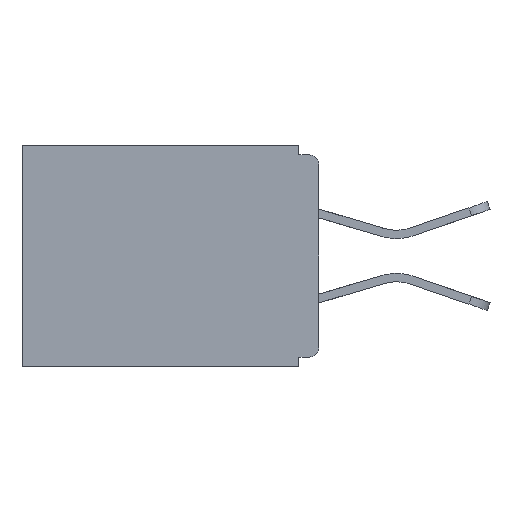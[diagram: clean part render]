
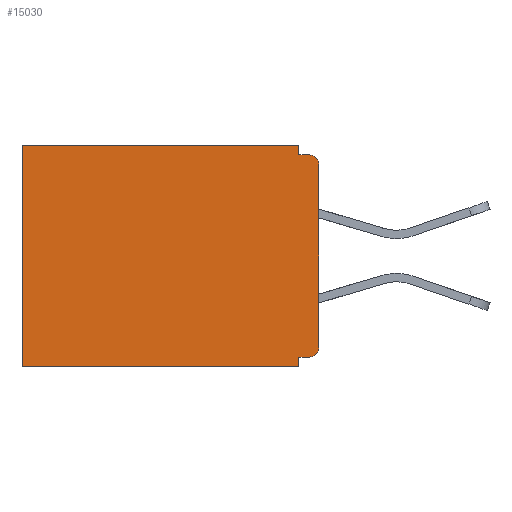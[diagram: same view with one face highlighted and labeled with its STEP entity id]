
A CAD part, left-side view. The second image highlights one B-rep face of the part: STEP entity #15030.
In plain terms, the highlighted planar face has unit normal (-1, 0, 0).
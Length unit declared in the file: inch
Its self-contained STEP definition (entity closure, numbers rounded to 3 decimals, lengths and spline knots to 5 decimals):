
#72 = VERTEX_POINT ( 'NONE', #19575 ) ;
#88 = DIRECTION ( 'NONE',  ( 0., 0., -1. ) ) ;
#672 = VECTOR ( 'NONE', #1396, 39.37008 ) ;
#871 = EDGE_CURVE ( 'NONE', #8522, #17490, #8414, .T. ) ;
#1396 = DIRECTION ( 'NONE',  ( 0., 0., -1. ) ) ;
#1463 = EDGE_CURVE ( 'NONE', #14093, #8041, #18573, .T. ) ;
#1473 = DIRECTION ( 'NONE',  ( 0., -1., 0. ) ) ;
#1577 = DIRECTION ( 'NONE',  ( 0., 0., -1. ) ) ;
#2273 = LINE ( 'NONE', #14384, #13811 ) ;
#2926 = EDGE_CURVE ( 'NONE', #14093, #8343, #18223, .T. ) ;
#3055 = ORIENTED_EDGE ( 'NONE', *, *, #6588, .T. ) ;
#3186 = VERTEX_POINT ( 'NONE', #16724 ) ;
#3974 = CARTESIAN_POINT ( 'NONE',  ( 0.298, 0.015, -0.328 ) ) ;
#4785 = ORIENTED_EDGE ( 'NONE', *, *, #9442, .F. ) ;
#4789 = DIRECTION ( 'NONE',  ( -1., 0., 0. ) ) ;
#4976 = CARTESIAN_POINT ( 'NONE',  ( 0.298, 0.031, -0.343 ) ) ;
#5769 = ORIENTED_EDGE ( 'NONE', *, *, #2926, .T. ) ;
#6076 = CARTESIAN_POINT ( 'NONE',  ( 0.298, 0., -0.328 ) ) ;
#6103 = CARTESIAN_POINT ( 'NONE',  ( 0.298, 0.015, -0.03 ) ) ;
#6588 = EDGE_CURVE ( 'NONE', #8075, #17490, #7877, .T. ) ;
#6614 = PLANE ( 'NONE',  #16510 ) ;
#6828 = ORIENTED_EDGE ( 'NONE', *, *, #19921, .T. ) ;
#6858 = LINE ( 'NONE', #13141, #7121 ) ;
#6919 = ORIENTED_EDGE ( 'NONE', *, *, #17527, .T. ) ;
#6967 = CARTESIAN_POINT ( 'NONE',  ( 0.298, 0., 0. ) ) ;
#7121 = VECTOR ( 'NONE', #1473, 39.37008 ) ;
#7652 = VERTEX_POINT ( 'NONE', #3974 ) ;
#7800 = DIRECTION ( 'NONE',  ( 0., 1., 0. ) ) ;
#7863 = VECTOR ( 'NONE', #19016, 39.37008 ) ;
#7877 = LINE ( 'NONE', #13534, #20760 ) ;
#8041 = VERTEX_POINT ( 'NONE', #13827 ) ;
#8075 = VERTEX_POINT ( 'NONE', #15954 ) ;
#8081 = CIRCLE ( 'NONE', #19873, 0.015 ) ;
#8231 = VECTOR ( 'NONE', #88, 39.37008 ) ;
#8343 = VERTEX_POINT ( 'NONE', #18941 ) ;
#8414 = LINE ( 'NONE', #17519, #7863 ) ;
#8522 = VERTEX_POINT ( 'NONE', #20768 ) ;
#9442 = EDGE_CURVE ( 'NONE', #9648, #8522, #17628, .T. ) ;
#9483 = LINE ( 'NONE', #6076, #13396 ) ;
#9648 = VERTEX_POINT ( 'NONE', #9981 ) ;
#9981 = CARTESIAN_POINT ( 'NONE',  ( 0.298, 0.031, -0.328 ) ) ;
#9983 = DIRECTION ( 'NONE',  ( 1., 0., 0. ) ) ;
#10261 = ORIENTED_EDGE ( 'NONE', *, *, #871, .F. ) ;
#10320 = EDGE_CURVE ( 'NONE', #7652, #9648, #9483, .T. ) ;
#10984 = ORIENTED_EDGE ( 'NONE', *, *, #16417, .F. ) ;
#11588 = FACE_OUTER_BOUND ( 'NONE', #12379, .T. ) ;
#11748 = CARTESIAN_POINT ( 'NONE',  ( 0.298, 0.015, -0.313 ) ) ;
#12283 = DIRECTION ( 'NONE',  ( 0., 0., -1. ) ) ;
#12379 = EDGE_LOOP ( 'NONE', ( #5769, #10984, #19087, #6919, #3055, #10261, #4785, #20620, #6828, #14695 ) ) ;
#12833 = DIRECTION ( 'NONE',  ( 0., 0., -1. ) ) ;
#13141 = CARTESIAN_POINT ( 'NONE',  ( 0.298, 0., -0.015 ) ) ;
#13396 = VECTOR ( 'NONE', #7800, 39.37008 ) ;
#13534 = CARTESIAN_POINT ( 'NONE',  ( 0.298, 0.46, 0. ) ) ;
#13811 = VECTOR ( 'NONE', #12833, 39.37008 ) ;
#13827 = CARTESIAN_POINT ( 'NONE',  ( 0.298, 0., -0.313 ) ) ;
#14093 = VERTEX_POINT ( 'NONE', #19792 ) ;
#14277 = AXIS2_PLACEMENT_3D ( 'NONE', #6103, #19577, #21236 ) ;
#14384 = CARTESIAN_POINT ( 'NONE',  ( 0.298, 0.031, -0.343 ) ) ;
#14695 = ORIENTED_EDGE ( 'NONE', *, *, #1463, .F. ) ;
#15030 = ADVANCED_FACE ( 'NONE', ( #11588 ), #6614, .F. ) ;
#15183 = LINE ( 'NONE', #6967, #21498 ) ;
#15310 = CARTESIAN_POINT ( 'NONE',  ( 0.298, 0.46, -0.343 ) ) ;
#15954 = CARTESIAN_POINT ( 'NONE',  ( 0.298, 0.46, 0. ) ) ;
#16344 = CARTESIAN_POINT ( 'NONE',  ( 0.298, 0., 0. ) ) ;
#16417 = EDGE_CURVE ( 'NONE', #72, #8343, #6858, .T. ) ;
#16510 = AXIS2_PLACEMENT_3D ( 'NONE', #18333, #9983, #1577 ) ;
#16539 = DIRECTION ( 'NONE',  ( 0., 0., -1. ) ) ;
#16724 = CARTESIAN_POINT ( 'NONE',  ( 0.298, 0.031, 0. ) ) ;
#17490 = VERTEX_POINT ( 'NONE', #15310 ) ;
#17519 = CARTESIAN_POINT ( 'NONE',  ( 0.298, 0., -0.343 ) ) ;
#17527 = EDGE_CURVE ( 'NONE', #3186, #8075, #15183, .T. ) ;
#17628 = LINE ( 'NONE', #4976, #8231 ) ;
#18223 = CIRCLE ( 'NONE', #14277, 0.015 ) ;
#18333 = CARTESIAN_POINT ( 'NONE',  ( 0.298, 0., 0. ) ) ;
#18515 = DIRECTION ( 'NONE',  ( 0., 1., 0. ) ) ;
#18573 = LINE ( 'NONE', #16344, #672 ) ;
#18758 = EDGE_CURVE ( 'NONE', #3186, #72, #2273, .T. ) ;
#18941 = CARTESIAN_POINT ( 'NONE',  ( 0.298, 0.015, -0.015 ) ) ;
#19016 = DIRECTION ( 'NONE',  ( 0., 1., 0. ) ) ;
#19087 = ORIENTED_EDGE ( 'NONE', *, *, #18758, .F. ) ;
#19575 = CARTESIAN_POINT ( 'NONE',  ( 0.298, 0.031, -0.015 ) ) ;
#19577 = DIRECTION ( 'NONE',  ( -1., 0., 0. ) ) ;
#19792 = CARTESIAN_POINT ( 'NONE',  ( 0.298, 0., -0.03 ) ) ;
#19873 = AXIS2_PLACEMENT_3D ( 'NONE', #11748, #4789, #16539 ) ;
#19921 = EDGE_CURVE ( 'NONE', #7652, #8041, #8081, .T. ) ;
#20620 = ORIENTED_EDGE ( 'NONE', *, *, #10320, .F. ) ;
#20760 = VECTOR ( 'NONE', #12283, 39.37008 ) ;
#20768 = CARTESIAN_POINT ( 'NONE',  ( 0.298, 0.031, -0.343 ) ) ;
#21236 = DIRECTION ( 'NONE',  ( 0., 0., -1. ) ) ;
#21498 = VECTOR ( 'NONE', #18515, 39.37008 ) ;
